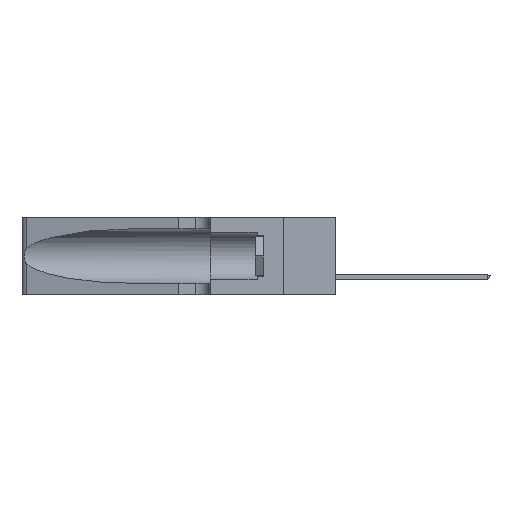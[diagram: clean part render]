
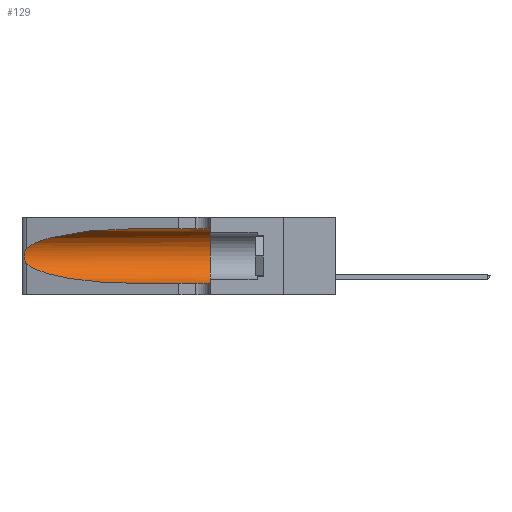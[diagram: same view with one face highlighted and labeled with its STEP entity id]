
A CAD part, left-side view. The second image highlights one B-rep face of the part: STEP entity #129.
In plain terms, the highlighted cylindrical face has radius 3.308 mm (diameter 6.617 mm), a partial arc.
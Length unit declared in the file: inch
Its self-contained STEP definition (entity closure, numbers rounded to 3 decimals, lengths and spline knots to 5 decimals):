
#129 = ADVANCED_FACE ( 'NONE', ( #3000 ), #3441, .F. ) ;
#442 = CARTESIAN_POINT ( 'NONE',  ( 0.25787, 1.23484, 0.2124 ) ) ;
#477 = AXIS2_PLACEMENT_3D ( 'NONE', #6306, #612, #11803 ) ;
#609 = CARTESIAN_POINT ( 'NONE',  ( 0.25639, 1.23186, 0.15144 ) ) ;
#612 = DIRECTION ( 'NONE',  ( 0., 1., 0. ) ) ;
#1168 = VERTEX_POINT ( 'NONE', #21431 ) ;
#1672 = CARTESIAN_POINT ( 'NONE',  ( 0.2373, 1.15595, 0.28018 ) ) ;
#1704 = VECTOR ( 'NONE', #24532, 39.37008 ) ;
#2149 = VERTEX_POINT ( 'NONE', #8321 ) ;
#2181 = CARTESIAN_POINT ( 'NONE',  ( 0.1305, 0.72297, 0.31525 ) ) ;
#2431 = CARTESIAN_POINT ( 'NONE',  ( 0.25639, 1.23184, 0.21858 ) ) ;
#3000 = FACE_OUTER_BOUND ( 'NONE', #5745, .T. ) ;
#3096 = CIRCLE ( 'NONE', #477, 0.13025 ) ;
#3441 = CYLINDRICAL_SURFACE ( 'NONE', #22000, 0.13025 ) ;
#4797 = CARTESIAN_POINT ( 'NONE',  ( 0.25487, 1.22718, 0.22369 ) ) ;
#5745 = EDGE_LOOP ( 'NONE', ( #23579, #11281, #16400, #37089, #17065, #9739 ) ) ;
#6306 = CARTESIAN_POINT ( 'NONE',  ( 0.1305, 0.35, 0.185 ) ) ;
#6455 = CARTESIAN_POINT ( 'NONE',  ( 0.1305, 1.61858, 0.31525 ) ) ;
#6802 = CARTESIAN_POINT ( 'NONE',  ( 0.26075, 1.23896, 0.178 ) ) ;
#7182 = CARTESIAN_POINT ( 'NONE',  ( 0.1305, 0.35, 0.05475 ) ) ;
#8165 = LINE ( 'NONE', #18889, #1704 ) ;
#8321 = CARTESIAN_POINT ( 'NONE',  ( 0.25487, 1.22718, 0.14631 ) ) ;
#9190 = DIRECTION ( 'NONE',  ( 0., -1., 0. ) ) ;
#9485 = CARTESIAN_POINT ( 'NONE',  ( 0.25856, 1.23593, 0.16098 ) ) ;
#9739 = ORIENTED_EDGE ( 'NONE', *, *, #28400, .F. ) ;
#10048 = CARTESIAN_POINT ( 'NONE',  ( 0.1305, 0.35, 0.31525 ) ) ;
#11281 = ORIENTED_EDGE ( 'NONE', *, *, #29714, .T. ) ;
#11803 = DIRECTION ( 'NONE',  ( 0., 0., 1. ) ) ;
#12255 = EDGE_CURVE ( 'NONE', #20455, #18528, #8165, .T. ) ;
#13352 = CARTESIAN_POINT ( 'NONE',  ( 0.1305, 0.72297, 0.31525 ) ) ;
#14093 = CARTESIAN_POINT ( 'NONE',  ( 0.26075, 1.23896, 0.19203 ) ) ;
#15371 = CARTESIAN_POINT ( 'NONE',  ( 0.26017, 1.23833, 0.17102 ) ) ;
#16400 = ORIENTED_EDGE ( 'NONE', *, *, #19851, .T. ) ;
#17065 = ORIENTED_EDGE ( 'NONE', *, *, #30287, .F. ) ;
#17131 = CARTESIAN_POINT ( 'NONE',  ( 0.25487, 1.22718, 0.14631 ) ) ;
#17988 = DIRECTION ( 'NONE',  ( 0., 0., -1. ) ) ;
#18435 = CARTESIAN_POINT ( 'NONE',  ( 0.25789, 1.23486, 0.15765 ) ) ;
#18528 = VERTEX_POINT ( 'NONE', #7182 ) ;
#18889 = CARTESIAN_POINT ( 'NONE',  ( 0.1305, 1.61858, 0.05475 ) ) ;
#19728 = CARTESIAN_POINT ( 'NONE',  ( 0.1305, 0.72297, 0.05475 ) ) ;
#19851 = EDGE_CURVE ( 'NONE', #2149, #20455, #31400, .T. ) ;
#20455 = VERTEX_POINT ( 'NONE', #19728 ) ;
#21431 = CARTESIAN_POINT ( 'NONE',  ( 0.25487, 1.22718, 0.22369 ) ) ;
#22000 = AXIS2_PLACEMENT_3D ( 'NONE', #26709, #9190, #17988 ) ;
#22278 = B_SPLINE_CURVE_WITH_KNOTS ( 'NONE', 3,
 ( #35967, #29590, #2431, #442, #34288, #33899, #14093, #6802, #15371, #9485, #18435, #609, #35814, #27263 ),
 .UNSPECIFIED., .F., .F.,
 ( 4, 2, 2, 2, 2, 2, 4 ),
 ( 0., 0.00027, 0.00053, 0.00107, 0.0016, 0.00187, 0.00214 ),
 .UNSPECIFIED. ) ;
#22661 = VERTEX_POINT ( 'NONE', #2181 ) ;
#23579 = ORIENTED_EDGE ( 'NONE', *, *, #34449, .T. ) ;
#24532 = DIRECTION ( 'NONE',  ( 0., -1., 0. ) ) ;
#24582 =( BOUNDED_CURVE ( )  B_SPLINE_CURVE ( 3, ( #13352, #28027, #1672, #4797 ),
 .UNSPECIFIED., .F., .F. ) 
 B_SPLINE_CURVE_WITH_KNOTS ( ( 4, 4 ),
 ( 1.5708, 2.84003 ),
 .UNSPECIFIED. ) 
 CURVE ( )  GEOMETRIC_REPRESENTATION_ITEM ( )  RATIONAL_B_SPLINE_CURVE ( ( 1., 0.87, 0.87, 1. ) ) 
 REPRESENTATION_ITEM ( '' )  );
#26560 = CARTESIAN_POINT ( 'NONE',  ( 0.1305, 0.72297, 0.05475 ) ) ;
#26709 = CARTESIAN_POINT ( 'NONE',  ( 0.1305, 1.61858, 0.185 ) ) ;
#27263 = CARTESIAN_POINT ( 'NONE',  ( 0.25487, 1.22718, 0.14631 ) ) ;
#28027 = CARTESIAN_POINT ( 'NONE',  ( 0.18966, 0.96281, 0.31525 ) ) ;
#28400 = EDGE_CURVE ( 'NONE', #22661, #30623, #35328, .T. ) ;
#29590 = CARTESIAN_POINT ( 'NONE',  ( 0.25555, 1.22994, 0.2215 ) ) ;
#29714 = EDGE_CURVE ( 'NONE', #1168, #2149, #22278, .T. ) ;
#30287 = EDGE_CURVE ( 'NONE', #30623, #18528, #3096, .T. ) ;
#30623 = VERTEX_POINT ( 'NONE', #10048 ) ;
#30727 = VECTOR ( 'NONE', #35722, 39.37008 ) ;
#31400 =( BOUNDED_CURVE ( )  B_SPLINE_CURVE ( 3, ( #17131, #34669, #32657, #26560 ),
 .UNSPECIFIED., .F., .T. ) 
 B_SPLINE_CURVE_WITH_KNOTS ( ( 4, 4 ),
 ( 3.44316, 4.71239 ),
 .UNSPECIFIED. ) 
 CURVE ( )  GEOMETRIC_REPRESENTATION_ITEM ( )  RATIONAL_B_SPLINE_CURVE ( ( 1., 0.87, 0.87, 1. ) ) 
 REPRESENTATION_ITEM ( '' )  );
#32657 = CARTESIAN_POINT ( 'NONE',  ( 0.18966, 0.96281, 0.05475 ) ) ;
#33899 = CARTESIAN_POINT ( 'NONE',  ( 0.26018, 1.23835, 0.19895 ) ) ;
#34288 = CARTESIAN_POINT ( 'NONE',  ( 0.25854, 1.2359, 0.20912 ) ) ;
#34449 = EDGE_CURVE ( 'NONE', #22661, #1168, #24582, .T. ) ;
#34669 = CARTESIAN_POINT ( 'NONE',  ( 0.2373, 1.15595, 0.08982 ) ) ;
#35328 = LINE ( 'NONE', #6455, #30727 ) ;
#35722 = DIRECTION ( 'NONE',  ( 0., -1., 0. ) ) ;
#35814 = CARTESIAN_POINT ( 'NONE',  ( 0.25555, 1.22993, 0.14849 ) ) ;
#35967 = CARTESIAN_POINT ( 'NONE',  ( 0.25487, 1.22718, 0.22369 ) ) ;
#37089 = ORIENTED_EDGE ( 'NONE', *, *, #12255, .T. ) ;
